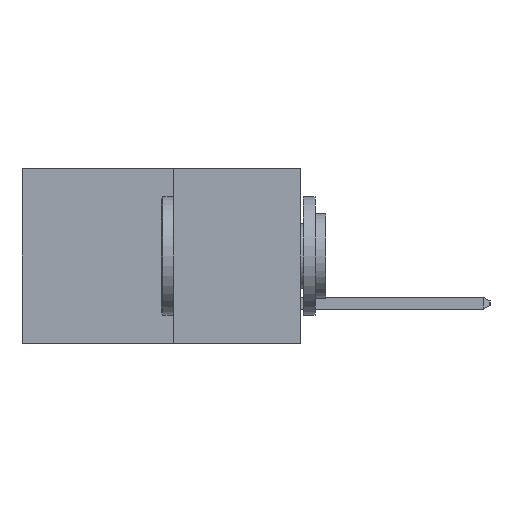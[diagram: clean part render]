
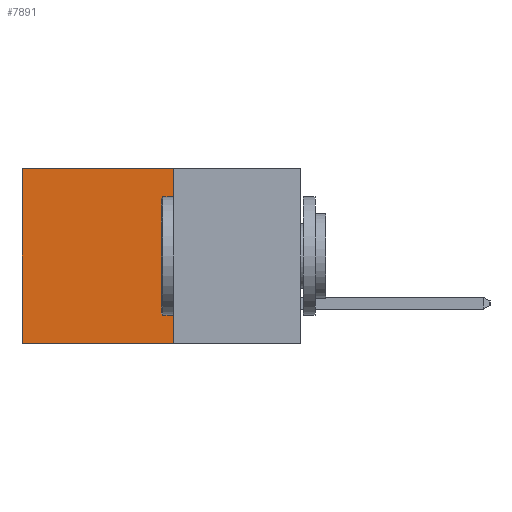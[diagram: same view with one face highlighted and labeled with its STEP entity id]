
A CAD part, left-side view. The second image highlights one B-rep face of the part: STEP entity #7891.
In plain terms, the highlighted planar face has unit normal (-1, 0, 0).
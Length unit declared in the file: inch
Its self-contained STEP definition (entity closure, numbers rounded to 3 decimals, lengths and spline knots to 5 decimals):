
#178 = CARTESIAN_POINT ( 'NONE',  ( 0.277, 0.27, 0. ) ) ;
#365 = CARTESIAN_POINT ( 'NONE',  ( 0.277, 0.59, 0. ) ) ;
#368 = VECTOR ( 'NONE', #6812, 39.37008 ) ;
#636 = CARTESIAN_POINT ( 'NONE',  ( 0.277, 0.27, -0.37 ) ) ;
#1239 = LINE ( 'NONE', #2028, #6357 ) ;
#1289 = EDGE_CURVE ( 'NONE', #6404, #8834, #4159, .T. ) ;
#1826 = CARTESIAN_POINT ( 'NONE',  ( 0.277, 0.59, -0.37 ) ) ;
#2028 = CARTESIAN_POINT ( 'NONE',  ( 0.277, 0.27, -0.37 ) ) ;
#2401 = DIRECTION ( 'NONE',  ( 0., 0., -1. ) ) ;
#2514 = PLANE ( 'NONE',  #7007 ) ;
#3302 = VERTEX_POINT ( 'NONE', #6506 ) ;
#3350 = ORIENTED_EDGE ( 'NONE', *, *, #5126, .F. ) ;
#3790 = ORIENTED_EDGE ( 'NONE', *, *, #1289, .T. ) ;
#3975 = EDGE_LOOP ( 'NONE', ( #4998, #3350, #5392, #3790 ) ) ;
#4071 = DIRECTION ( 'NONE',  ( 0., 0., -1. ) ) ;
#4159 = LINE ( 'NONE', #178, #368 ) ;
#4190 = DIRECTION ( 'NONE',  ( 1., 0., 0. ) ) ;
#4681 = VECTOR ( 'NONE', #6459, 39.37008 ) ;
#4981 = VERTEX_POINT ( 'NONE', #6610 ) ;
#4998 = ORIENTED_EDGE ( 'NONE', *, *, #7652, .T. ) ;
#5005 = CARTESIAN_POINT ( 'NONE',  ( 0.277, 0.27, 0. ) ) ;
#5126 = EDGE_CURVE ( 'NONE', #4981, #3302, #1239, .T. ) ;
#5387 = LINE ( 'NONE', #1826, #8625 ) ;
#5392 = ORIENTED_EDGE ( 'NONE', *, *, #6250, .F. ) ;
#5471 = DIRECTION ( 'NONE',  ( 0., 1., 0. ) ) ;
#6250 = EDGE_CURVE ( 'NONE', #6404, #4981, #8146, .T. ) ;
#6357 = VECTOR ( 'NONE', #5471, 39.37008 ) ;
#6404 = VERTEX_POINT ( 'NONE', #5005 ) ;
#6459 = DIRECTION ( 'NONE',  ( 0., 0., -1. ) ) ;
#6506 = CARTESIAN_POINT ( 'NONE',  ( 0.277, 0.59, -0.37 ) ) ;
#6610 = CARTESIAN_POINT ( 'NONE',  ( 0.277, 0.27, -0.37 ) ) ;
#6812 = DIRECTION ( 'NONE',  ( 0., 1., 0. ) ) ;
#7007 = AXIS2_PLACEMENT_3D ( 'NONE', #636, #4190, #4071 ) ;
#7152 = CARTESIAN_POINT ( 'NONE',  ( 0.277, 0.27, -0.37 ) ) ;
#7652 = EDGE_CURVE ( 'NONE', #8834, #3302, #5387, .T. ) ;
#7891 = ADVANCED_FACE ( 'NONE', ( #8520 ), #2514, .F. ) ;
#8146 = LINE ( 'NONE', #7152, #4681 ) ;
#8520 = FACE_OUTER_BOUND ( 'NONE', #3975, .T. ) ;
#8625 = VECTOR ( 'NONE', #2401, 39.37008 ) ;
#8834 = VERTEX_POINT ( 'NONE', #365 ) ;
